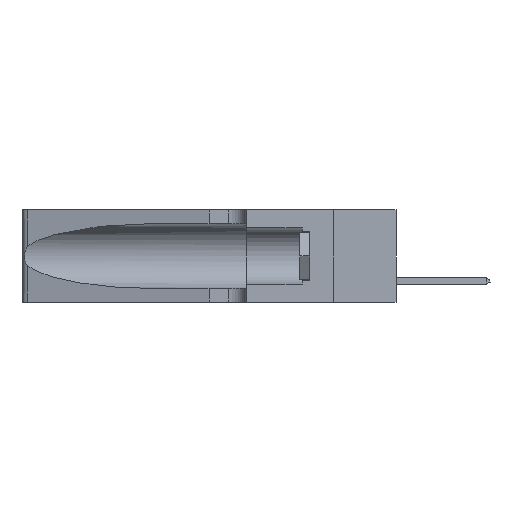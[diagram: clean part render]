
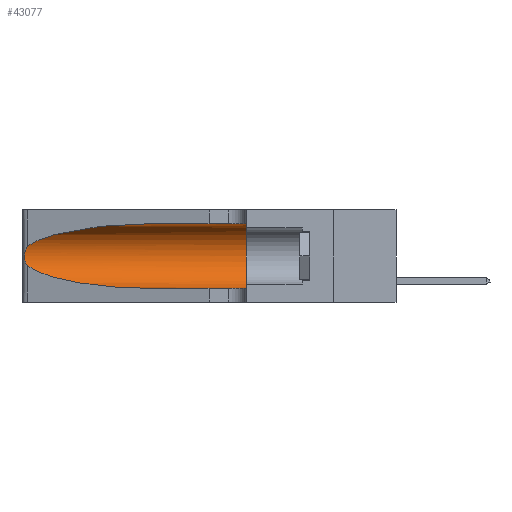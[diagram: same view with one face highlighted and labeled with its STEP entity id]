
A CAD part, left-side view. The second image highlights one B-rep face of the part: STEP entity #43077.
In plain terms, the highlighted cylindrical face has radius 3.308 mm (diameter 6.617 mm), a partial arc.
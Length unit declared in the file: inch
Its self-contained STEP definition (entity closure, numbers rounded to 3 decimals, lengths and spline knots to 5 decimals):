
#1628 = CARTESIAN_POINT ( 'NONE',  ( 0.18966, 0.96281, 0.05475 ) ) ;
#1845 = EDGE_CURVE ( 'NONE', #22982, #20328, #22392, .T. ) ;
#2055 = CARTESIAN_POINT ( 'NONE',  ( 0.25487, 1.22718, 0.14631 ) ) ;
#2106 = EDGE_CURVE ( 'NONE', #20328, #8189, #40869, .T. ) ;
#2304 = CARTESIAN_POINT ( 'NONE',  ( 0.1305, 0.72297, 0.31525 ) ) ;
#3189 =( BOUNDED_CURVE ( )  B_SPLINE_CURVE ( 3, ( #2304, #21629, #26347, #13878 ),
 .UNSPECIFIED., .F., .F. ) 
 B_SPLINE_CURVE_WITH_KNOTS ( ( 4, 4 ),
 ( 1.5708, 2.84003 ),
 .UNSPECIFIED. ) 
 CURVE ( )  GEOMETRIC_REPRESENTATION_ITEM ( )  RATIONAL_B_SPLINE_CURVE ( ( 1., 0.87, 0.87, 1. ) ) 
 REPRESENTATION_ITEM ( '' )  );
#3540 = ORIENTED_EDGE ( 'NONE', *, *, #49438, .T. ) ;
#5134 = DIRECTION ( 'NONE',  ( 0., 0., -1. ) ) ;
#7081 = CARTESIAN_POINT ( 'NONE',  ( 0.25854, 1.2359, 0.20912 ) ) ;
#7269 = CARTESIAN_POINT ( 'NONE',  ( 0.25787, 1.23484, 0.2124 ) ) ;
#8189 = VERTEX_POINT ( 'NONE', #41055 ) ;
#8533 = ORIENTED_EDGE ( 'NONE', *, *, #22608, .T. ) ;
#9383 = CARTESIAN_POINT ( 'NONE',  ( 0.1305, 0.72297, 0.31525 ) ) ;
#9931 = AXIS2_PLACEMENT_3D ( 'NONE', #28300, #48394, #5134 ) ;
#10646 = CARTESIAN_POINT ( 'NONE',  ( 0.25639, 1.23184, 0.21858 ) ) ;
#10799 = B_SPLINE_CURVE_WITH_KNOTS ( 'NONE', 3,
 ( #26543, #10838, #10646, #7269, #7081, #50506, #38296, #14810, #42438, #22726, #26901, #46496, #42611, #14447 ),
 .UNSPECIFIED., .F., .F.,
 ( 4, 2, 2, 2, 2, 2, 4 ),
 ( 0., 0.00027, 0.00053, 0.00107, 0.0016, 0.00187, 0.00214 ),
 .UNSPECIFIED. ) ;
#10838 = CARTESIAN_POINT ( 'NONE',  ( 0.25555, 1.22994, 0.2215 ) ) ;
#11908 = VECTOR ( 'NONE', #22934, 39.37008 ) ;
#12791 = ORIENTED_EDGE ( 'NONE', *, *, #1845, .F. ) ;
#13878 = CARTESIAN_POINT ( 'NONE',  ( 0.25487, 1.22718, 0.22369 ) ) ;
#14168 = CARTESIAN_POINT ( 'NONE',  ( 0.1305, 0.72297, 0.05475 ) ) ;
#14447 = CARTESIAN_POINT ( 'NONE',  ( 0.25487, 1.22718, 0.14631 ) ) ;
#14810 = CARTESIAN_POINT ( 'NONE',  ( 0.26075, 1.23896, 0.178 ) ) ;
#15913 = ORIENTED_EDGE ( 'NONE', *, *, #44327, .T. ) ;
#18051 = CARTESIAN_POINT ( 'NONE',  ( 0.2373, 1.15595, 0.08982 ) ) ;
#18925 = FACE_OUTER_BOUND ( 'NONE', #40352, .T. ) ;
#19317 =( BOUNDED_CURVE ( )  B_SPLINE_CURVE ( 3, ( #27450, #18051, #1628, #14168 ),
 .UNSPECIFIED., .F., .T. ) 
 B_SPLINE_CURVE_WITH_KNOTS ( ( 4, 4 ),
 ( 3.44316, 4.71239 ),
 .UNSPECIFIED. ) 
 CURVE ( )  GEOMETRIC_REPRESENTATION_ITEM ( )  RATIONAL_B_SPLINE_CURVE ( ( 1., 0.87, 0.87, 1. ) ) 
 REPRESENTATION_ITEM ( '' )  );
#20328 = VERTEX_POINT ( 'NONE', #24495 ) ;
#21629 = CARTESIAN_POINT ( 'NONE',  ( 0.18966, 0.96281, 0.31525 ) ) ;
#21745 = VERTEX_POINT ( 'NONE', #43482 ) ;
#22392 = LINE ( 'NONE', #30722, #11908 ) ;
#22478 = VECTOR ( 'NONE', #43195, 39.37008 ) ;
#22608 = EDGE_CURVE ( 'NONE', #22982, #21745, #3189, .T. ) ;
#22726 = CARTESIAN_POINT ( 'NONE',  ( 0.25856, 1.23593, 0.16098 ) ) ;
#22934 = DIRECTION ( 'NONE',  ( 0., -1., 0. ) ) ;
#22982 = VERTEX_POINT ( 'NONE', #9383 ) ;
#23326 = DIRECTION ( 'NONE',  ( 0., 0., 1. ) ) ;
#24495 = CARTESIAN_POINT ( 'NONE',  ( 0.1305, 0.35, 0.31525 ) ) ;
#25811 = VERTEX_POINT ( 'NONE', #31169 ) ;
#26029 = AXIS2_PLACEMENT_3D ( 'NONE', #39214, #50409, #23326 ) ;
#26340 = CYLINDRICAL_SURFACE ( 'NONE', #9931, 0.13025 ) ;
#26347 = CARTESIAN_POINT ( 'NONE',  ( 0.2373, 1.15595, 0.28018 ) ) ;
#26543 = CARTESIAN_POINT ( 'NONE',  ( 0.25487, 1.22718, 0.22369 ) ) ;
#26901 = CARTESIAN_POINT ( 'NONE',  ( 0.25789, 1.23486, 0.15765 ) ) ;
#27450 = CARTESIAN_POINT ( 'NONE',  ( 0.25487, 1.22718, 0.14631 ) ) ;
#28300 = CARTESIAN_POINT ( 'NONE',  ( 0.1305, 1.61858, 0.185 ) ) ;
#30298 = ORIENTED_EDGE ( 'NONE', *, *, #2106, .F. ) ;
#30722 = CARTESIAN_POINT ( 'NONE',  ( 0.1305, 1.61858, 0.31525 ) ) ;
#31169 = CARTESIAN_POINT ( 'NONE',  ( 0.1305, 0.72297, 0.05475 ) ) ;
#33529 = LINE ( 'NONE', #35749, #22478 ) ;
#35749 = CARTESIAN_POINT ( 'NONE',  ( 0.1305, 1.61858, 0.05475 ) ) ;
#38296 = CARTESIAN_POINT ( 'NONE',  ( 0.26075, 1.23896, 0.19203 ) ) ;
#39214 = CARTESIAN_POINT ( 'NONE',  ( 0.1305, 0.35, 0.185 ) ) ;
#39606 = EDGE_CURVE ( 'NONE', #21745, #40062, #10799, .T. ) ;
#40062 = VERTEX_POINT ( 'NONE', #2055 ) ;
#40352 = EDGE_LOOP ( 'NONE', ( #8533, #42873, #3540, #15913, #30298, #12791 ) ) ;
#40869 = CIRCLE ( 'NONE', #26029, 0.13025 ) ;
#41055 = CARTESIAN_POINT ( 'NONE',  ( 0.1305, 0.35, 0.05475 ) ) ;
#42438 = CARTESIAN_POINT ( 'NONE',  ( 0.26017, 1.23833, 0.17102 ) ) ;
#42611 = CARTESIAN_POINT ( 'NONE',  ( 0.25555, 1.22993, 0.14849 ) ) ;
#42873 = ORIENTED_EDGE ( 'NONE', *, *, #39606, .T. ) ;
#43077 = ADVANCED_FACE ( 'NONE', ( #18925 ), #26340, .F. ) ;
#43195 = DIRECTION ( 'NONE',  ( 0., -1., 0. ) ) ;
#43482 = CARTESIAN_POINT ( 'NONE',  ( 0.25487, 1.22718, 0.22369 ) ) ;
#44327 = EDGE_CURVE ( 'NONE', #25811, #8189, #33529, .T. ) ;
#46496 = CARTESIAN_POINT ( 'NONE',  ( 0.25639, 1.23186, 0.15144 ) ) ;
#48394 = DIRECTION ( 'NONE',  ( 0., -1., 0. ) ) ;
#49438 = EDGE_CURVE ( 'NONE', #40062, #25811, #19317, .T. ) ;
#50409 = DIRECTION ( 'NONE',  ( 0., 1., 0. ) ) ;
#50506 = CARTESIAN_POINT ( 'NONE',  ( 0.26018, 1.23835, 0.19895 ) ) ;
